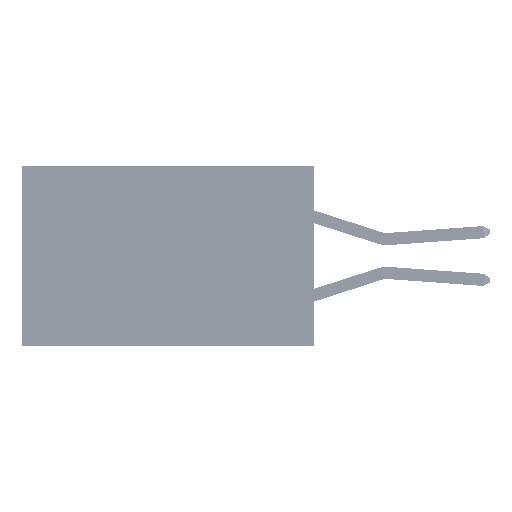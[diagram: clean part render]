
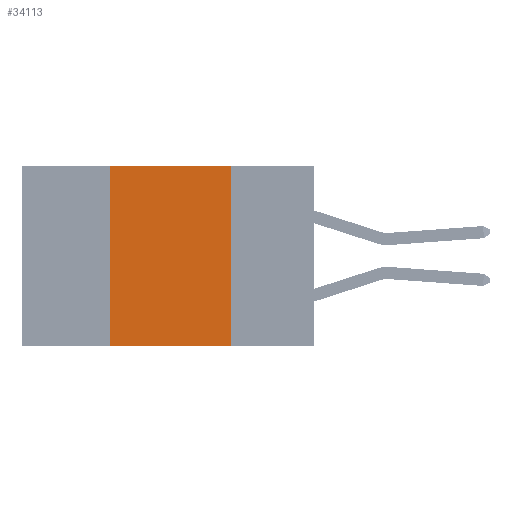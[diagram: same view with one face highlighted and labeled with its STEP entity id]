
A CAD part, left-side view. The second image highlights one B-rep face of the part: STEP entity #34113.
In plain terms, the highlighted planar face has unit normal (-1, 0, 0).
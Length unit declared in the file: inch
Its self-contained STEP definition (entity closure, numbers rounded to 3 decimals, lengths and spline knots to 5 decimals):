
#2093 = ORIENTED_EDGE ( 'NONE', *, *, #2814, .T. ) ;
#2814 = EDGE_CURVE ( 'NONE', #4275, #47763, #32021, .T. ) ;
#4275 = VERTEX_POINT ( 'NONE', #17639 ) ;
#5432 = CARTESIAN_POINT ( 'NONE',  ( 0., 0.6, 0. ) ) ;
#6993 = VECTOR ( 'NONE', #28041, 39.37008 ) ;
#7692 = VERTEX_POINT ( 'NONE', #16768 ) ;
#9650 = AXIS2_PLACEMENT_3D ( 'NONE', #36367, #17431, #28147 ) ;
#11808 = DIRECTION ( 'NONE',  ( 0., 0., 1. ) ) ;
#13485 = LINE ( 'NONE', #42898, #16729 ) ;
#16729 = VECTOR ( 'NONE', #39660, 39.37008 ) ;
#16768 = CARTESIAN_POINT ( 'NONE',  ( 0., 0.17, 0. ) ) ;
#17431 = DIRECTION ( 'NONE',  ( 1., 0., 0. ) ) ;
#17639 = CARTESIAN_POINT ( 'NONE',  ( 0., 0.42, -0.37 ) ) ;
#18272 = ORIENTED_EDGE ( 'NONE', *, *, #28215, .F. ) ;
#20377 = DIRECTION ( 'NONE',  ( 0., -1., 0. ) ) ;
#22388 = VERTEX_POINT ( 'NONE', #28455 ) ;
#26766 = VECTOR ( 'NONE', #11808, 39.37008 ) ;
#27756 = ORIENTED_EDGE ( 'NONE', *, *, #34434, .F. ) ;
#28041 = DIRECTION ( 'NONE',  ( 0., -1., 0. ) ) ;
#28147 = DIRECTION ( 'NONE',  ( 0., 0., -1. ) ) ;
#28215 = EDGE_CURVE ( 'NONE', #4275, #22388, #45954, .T. ) ;
#28455 = CARTESIAN_POINT ( 'NONE',  ( 0., 0.42, 0. ) ) ;
#31881 = PLANE ( 'NONE',  #9650 ) ;
#32021 = LINE ( 'NONE', #39278, #6993 ) ;
#33584 = EDGE_LOOP ( 'NONE', ( #39301, #27756, #18272, #2093 ) ) ;
#34113 = ADVANCED_FACE ( 'NONE', ( #40131 ), #31881, .F. ) ;
#34434 = EDGE_CURVE ( 'NONE', #22388, #7692, #39083, .T. ) ;
#36367 = CARTESIAN_POINT ( 'NONE',  ( 0., 0.6, 0. ) ) ;
#36868 = CARTESIAN_POINT ( 'NONE',  ( 0., 0.17, -0.37 ) ) ;
#39083 = LINE ( 'NONE', #5432, #46197 ) ;
#39278 = CARTESIAN_POINT ( 'NONE',  ( 0., 0.6, -0.37 ) ) ;
#39301 = ORIENTED_EDGE ( 'NONE', *, *, #39834, .F. ) ;
#39660 = DIRECTION ( 'NONE',  ( 0., 0., -1. ) ) ;
#39834 = EDGE_CURVE ( 'NONE', #7692, #47763, #13485, .T. ) ;
#40131 = FACE_OUTER_BOUND ( 'NONE', #33584, .T. ) ;
#42898 = CARTESIAN_POINT ( 'NONE',  ( 0., 0.17, 0. ) ) ;
#45954 = LINE ( 'NONE', #46445, #26766 ) ;
#46197 = VECTOR ( 'NONE', #20377, 39.37008 ) ;
#46445 = CARTESIAN_POINT ( 'NONE',  ( 0., 0.42, 0. ) ) ;
#47763 = VERTEX_POINT ( 'NONE', #36868 ) ;
